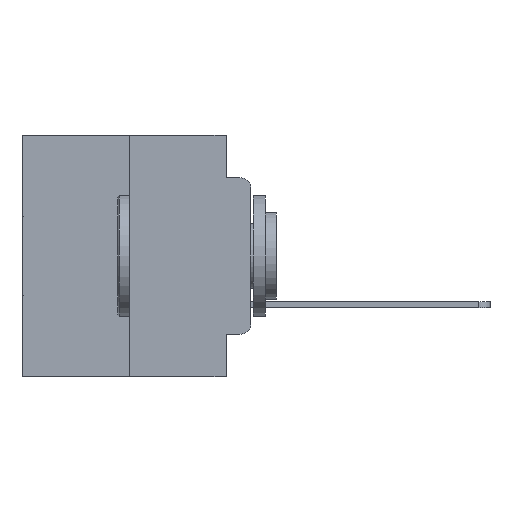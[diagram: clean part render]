
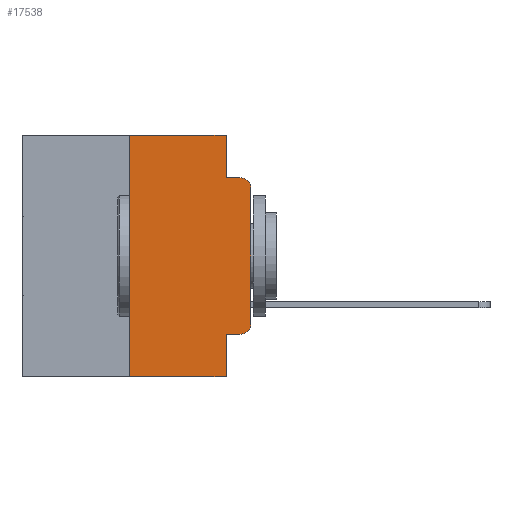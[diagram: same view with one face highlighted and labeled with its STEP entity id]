
A CAD part, left-side view. The second image highlights one B-rep face of the part: STEP entity #17538.
In plain terms, the highlighted planar face has unit normal (-1, 0, 0).
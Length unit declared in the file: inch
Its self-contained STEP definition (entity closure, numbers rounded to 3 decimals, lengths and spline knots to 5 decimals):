
#80 = VERTEX_POINT ( 'NONE', #17363 ) ;
#224 = ORIENTED_EDGE ( 'NONE', *, *, #26473, .F. ) ;
#287 = DIRECTION ( 'NONE',  ( 0., -1., 0. ) ) ;
#1102 = DIRECTION ( 'NONE',  ( 1., 0., 0. ) ) ;
#1271 = DIRECTION ( 'NONE',  ( 0., -1., 0. ) ) ;
#1412 = ORIENTED_EDGE ( 'NONE', *, *, #7578, .T. ) ;
#2375 = ORIENTED_EDGE ( 'NONE', *, *, #6962, .F. ) ;
#2555 = CARTESIAN_POINT ( 'NONE',  ( 0., 0., -0.3915 ) ) ;
#2690 = CARTESIAN_POINT ( 'NONE',  ( 0., 0.02, -0.1085 ) ) ;
#2911 = VECTOR ( 'NONE', #28389, 39.37008 ) ;
#2925 = DIRECTION ( 'NONE',  ( -1., 0., 0. ) ) ;
#3414 = AXIS2_PLACEMENT_3D ( 'NONE', #17815, #2925, #20103 ) ;
#3461 = VERTEX_POINT ( 'NONE', #29042 ) ;
#4080 = VERTEX_POINT ( 'NONE', #10696 ) ;
#4165 = CARTESIAN_POINT ( 'NONE',  ( 0., 0.02, -0.0885 ) ) ;
#4413 = CARTESIAN_POINT ( 'NONE',  ( 0., 0.051, 0. ) ) ;
#4453 = AXIS2_PLACEMENT_3D ( 'NONE', #2690, #19907, #5448 ) ;
#4666 = CARTESIAN_POINT ( 'NONE',  ( 0., 0.25, 0. ) ) ;
#4837 = VECTOR ( 'NONE', #287, 39.37008 ) ;
#5197 = EDGE_CURVE ( 'NONE', #6678, #80, #14660, .T. ) ;
#5262 = ORIENTED_EDGE ( 'NONE', *, *, #22866, .T. ) ;
#5448 = DIRECTION ( 'NONE',  ( 0., 0., -1. ) ) ;
#5944 = EDGE_CURVE ( 'NONE', #20044, #28242, #28254, .T. ) ;
#6041 = ORIENTED_EDGE ( 'NONE', *, *, #5197, .F. ) ;
#6678 = VERTEX_POINT ( 'NONE', #4413 ) ;
#6831 = DIRECTION ( 'NONE',  ( 0., 0., 1. ) ) ;
#6923 = LINE ( 'NONE', #18832, #12658 ) ;
#6962 = EDGE_CURVE ( 'NONE', #80, #25232, #12271, .T. ) ;
#7578 = EDGE_CURVE ( 'NONE', #18908, #17863, #26389, .T. ) ;
#7601 = CARTESIAN_POINT ( 'NONE',  ( 0., 0.02, -0.4115 ) ) ;
#7724 = ORIENTED_EDGE ( 'NONE', *, *, #15103, .T. ) ;
#8964 = VECTOR ( 'NONE', #1271, 39.37008 ) ;
#9836 = LINE ( 'NONE', #4666, #2911 ) ;
#10574 = CARTESIAN_POINT ( 'NONE',  ( 0., 0.25, 0. ) ) ;
#10657 = CARTESIAN_POINT ( 'NONE',  ( 0., 0.051, -0.0885 ) ) ;
#10696 = CARTESIAN_POINT ( 'NONE',  ( 0., 0.051, -0.4115 ) ) ;
#11723 = DIRECTION ( 'NONE',  ( 0., 0., -1. ) ) ;
#12271 = LINE ( 'NONE', #10657, #4837 ) ;
#12647 = VECTOR ( 'NONE', #11723, 39.37008 ) ;
#12658 = VECTOR ( 'NONE', #6831, 39.37008 ) ;
#13185 = ORIENTED_EDGE ( 'NONE', *, *, #14120, .T. ) ;
#13390 = EDGE_CURVE ( 'NONE', #24919, #6678, #17362, .T. ) ;
#14120 = EDGE_CURVE ( 'NONE', #4080, #18908, #17688, .T. ) ;
#14660 = LINE ( 'NONE', #15626, #25490 ) ;
#15103 = EDGE_CURVE ( 'NONE', #3461, #25232, #16899, .T. ) ;
#15399 = ORIENTED_EDGE ( 'NONE', *, *, #27996, .F. ) ;
#15626 = CARTESIAN_POINT ( 'NONE',  ( 0., 0.051, 0. ) ) ;
#16227 = CARTESIAN_POINT ( 'NONE',  ( 0., 0.473, 0. ) ) ;
#16899 = CIRCLE ( 'NONE', #4453, 0.02 ) ;
#17323 = ORIENTED_EDGE ( 'NONE', *, *, #5944, .T. ) ;
#17362 = LINE ( 'NONE', #23608, #22734 ) ;
#17363 = CARTESIAN_POINT ( 'NONE',  ( 0., 0.051, -0.0885 ) ) ;
#17538 = ADVANCED_FACE ( 'NONE', ( #24738 ), #25349, .F. ) ;
#17688 = LINE ( 'NONE', #28107, #23047 ) ;
#17815 = CARTESIAN_POINT ( 'NONE',  ( 0., 0.02, -0.3915 ) ) ;
#17863 = VERTEX_POINT ( 'NONE', #2555 ) ;
#17965 = CARTESIAN_POINT ( 'NONE',  ( 0., 0.051, -0.5 ) ) ;
#18131 = DIRECTION ( 'NONE',  ( 0., 0., -1. ) ) ;
#18576 = DIRECTION ( 'NONE',  ( 0., 0., -1. ) ) ;
#18792 = CARTESIAN_POINT ( 'NONE',  ( 0., 0.051, 0. ) ) ;
#18832 = CARTESIAN_POINT ( 'NONE',  ( 0., 0., 0. ) ) ;
#18908 = VERTEX_POINT ( 'NONE', #7601 ) ;
#18953 = LINE ( 'NONE', #18792, #12647 ) ;
#19907 = DIRECTION ( 'NONE',  ( -1., 0., 0. ) ) ;
#20044 = VERTEX_POINT ( 'NONE', #30103 ) ;
#20103 = DIRECTION ( 'NONE',  ( 0., 0., -1. ) ) ;
#22734 = VECTOR ( 'NONE', #28130, 39.37008 ) ;
#22866 = EDGE_CURVE ( 'NONE', #17863, #3461, #6923, .T. ) ;
#23047 = VECTOR ( 'NONE', #23676, 39.37008 ) ;
#23608 = CARTESIAN_POINT ( 'NONE',  ( 0., 0.473, 0. ) ) ;
#23676 = DIRECTION ( 'NONE',  ( 0., -1., 0. ) ) ;
#23975 = EDGE_LOOP ( 'NONE', ( #5262, #7724, #2375, #6041, #29153, #15399, #17323, #224, #13185, #1412 ) ) ;
#24738 = FACE_OUTER_BOUND ( 'NONE', #23975, .T. ) ;
#24919 = VERTEX_POINT ( 'NONE', #10574 ) ;
#25232 = VERTEX_POINT ( 'NONE', #4165 ) ;
#25349 = PLANE ( 'NONE',  #28703 ) ;
#25484 = CARTESIAN_POINT ( 'NONE',  ( 0., 0.473, -0.5 ) ) ;
#25490 = VECTOR ( 'NONE', #18131, 39.37008 ) ;
#26389 = CIRCLE ( 'NONE', #3414, 0.02 ) ;
#26473 = EDGE_CURVE ( 'NONE', #4080, #28242, #18953, .T. ) ;
#27996 = EDGE_CURVE ( 'NONE', #20044, #24919, #9836, .T. ) ;
#28107 = CARTESIAN_POINT ( 'NONE',  ( 0., 0.051, -0.4115 ) ) ;
#28130 = DIRECTION ( 'NONE',  ( 0., -1., 0. ) ) ;
#28242 = VERTEX_POINT ( 'NONE', #17965 ) ;
#28254 = LINE ( 'NONE', #25484, #8964 ) ;
#28389 = DIRECTION ( 'NONE',  ( 0., 0., 1. ) ) ;
#28703 = AXIS2_PLACEMENT_3D ( 'NONE', #16227, #1102, #18576 ) ;
#29042 = CARTESIAN_POINT ( 'NONE',  ( 0., 0., -0.1085 ) ) ;
#29153 = ORIENTED_EDGE ( 'NONE', *, *, #13390, .F. ) ;
#30103 = CARTESIAN_POINT ( 'NONE',  ( 0., 0.25, -0.5 ) ) ;
